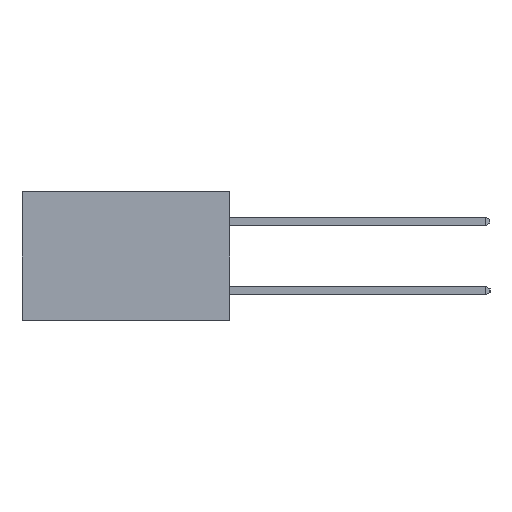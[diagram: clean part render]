
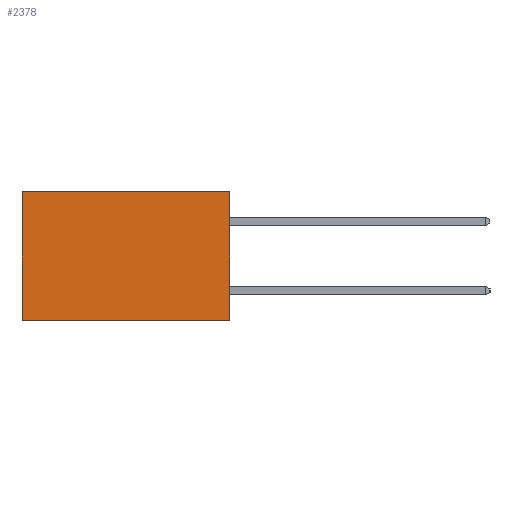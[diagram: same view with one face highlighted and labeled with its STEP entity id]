
A CAD part, left-side view. The second image highlights one B-rep face of the part: STEP entity #2378.
In plain terms, the highlighted planar face has unit normal (-1, 0, 0).
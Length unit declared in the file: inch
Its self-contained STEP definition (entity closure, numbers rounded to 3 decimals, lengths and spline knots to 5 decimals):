
#76 = LINE ( 'NONE', #12915, #2851 ) ;
#493 = VECTOR ( 'NONE', #6012, 39.37008 ) ;
#822 = VECTOR ( 'NONE', #14275, 39.37008 ) ;
#996 = ORIENTED_EDGE ( 'NONE', *, *, #8088, .T. ) ;
#1178 = EDGE_CURVE ( 'NONE', #8995, #1229, #76, .T. ) ;
#1229 = VERTEX_POINT ( 'NONE', #8463 ) ;
#1484 = VERTEX_POINT ( 'NONE', #2190 ) ;
#1714 = CARTESIAN_POINT ( 'NONE',  ( 0.2615, 0.6, 0. ) ) ;
#1790 = DIRECTION ( 'NONE',  ( 0., 0., -1. ) ) ;
#2140 = EDGE_LOOP ( 'NONE', ( #11184, #11924, #2664, #996 ) ) ;
#2190 = CARTESIAN_POINT ( 'NONE',  ( 0.2615, 0.6, -0.37 ) ) ;
#2378 = ADVANCED_FACE ( 'NONE', ( #12766 ), #3359, .F. ) ;
#2664 = ORIENTED_EDGE ( 'NONE', *, *, #1178, .F. ) ;
#2851 = VECTOR ( 'NONE', #1790, 39.37008 ) ;
#3359 = PLANE ( 'NONE',  #10655 ) ;
#3596 = LINE ( 'NONE', #11804, #493 ) ;
#5036 = CARTESIAN_POINT ( 'NONE',  ( 0.2615, 0., -0.37 ) ) ;
#5399 = EDGE_CURVE ( 'NONE', #1229, #1484, #10303, .T. ) ;
#6012 = DIRECTION ( 'NONE',  ( 0., 1., 0. ) ) ;
#6843 = DIRECTION ( 'NONE',  ( 0., 1., 0. ) ) ;
#7056 = LINE ( 'NONE', #9700, #822 ) ;
#8004 = CARTESIAN_POINT ( 'NONE',  ( 0.2615, 0., -0.37 ) ) ;
#8088 = EDGE_CURVE ( 'NONE', #8995, #11482, #3596, .T. ) ;
#8463 = CARTESIAN_POINT ( 'NONE',  ( 0.2615, 0., -0.37 ) ) ;
#8995 = VERTEX_POINT ( 'NONE', #10862 ) ;
#9013 = EDGE_CURVE ( 'NONE', #11482, #1484, #7056, .T. ) ;
#9700 = CARTESIAN_POINT ( 'NONE',  ( 0.2615, 0.6, -0.37 ) ) ;
#9966 = DIRECTION ( 'NONE',  ( 0., 0., -1. ) ) ;
#10303 = LINE ( 'NONE', #8004, #12963 ) ;
#10655 = AXIS2_PLACEMENT_3D ( 'NONE', #5036, #11398, #9966 ) ;
#10862 = CARTESIAN_POINT ( 'NONE',  ( 0.2615, 0., 0. ) ) ;
#11184 = ORIENTED_EDGE ( 'NONE', *, *, #9013, .T. ) ;
#11398 = DIRECTION ( 'NONE',  ( 1., 0., 0. ) ) ;
#11482 = VERTEX_POINT ( 'NONE', #1714 ) ;
#11804 = CARTESIAN_POINT ( 'NONE',  ( 0.2615, 0., 0. ) ) ;
#11924 = ORIENTED_EDGE ( 'NONE', *, *, #5399, .F. ) ;
#12766 = FACE_OUTER_BOUND ( 'NONE', #2140, .T. ) ;
#12915 = CARTESIAN_POINT ( 'NONE',  ( 0.2615, 0., -0.37 ) ) ;
#12963 = VECTOR ( 'NONE', #6843, 39.37008 ) ;
#14275 = DIRECTION ( 'NONE',  ( 0., 0., -1. ) ) ;
